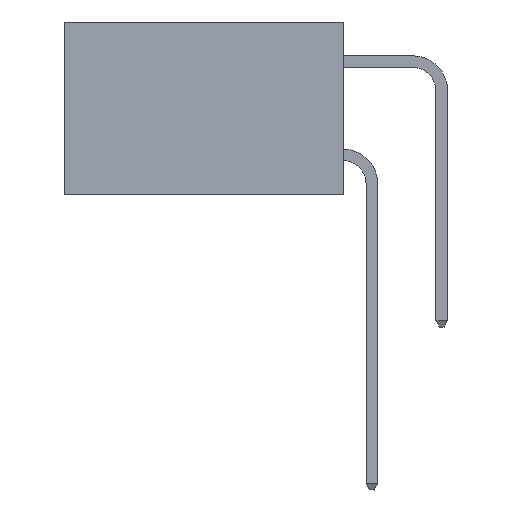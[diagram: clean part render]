
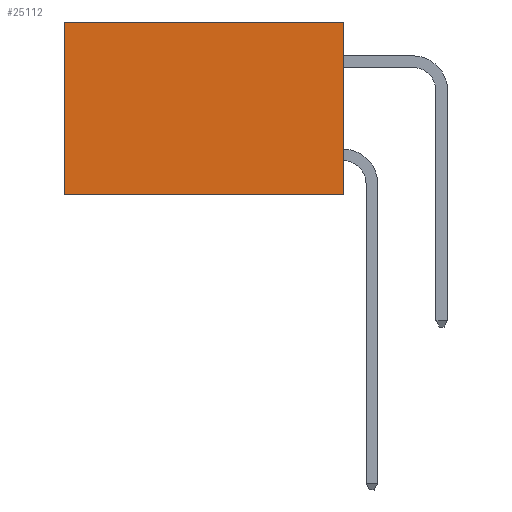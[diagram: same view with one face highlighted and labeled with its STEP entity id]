
A CAD part, left-side view. The second image highlights one B-rep face of the part: STEP entity #25112.
In plain terms, the highlighted planar face has unit normal (-1, 0, 0).
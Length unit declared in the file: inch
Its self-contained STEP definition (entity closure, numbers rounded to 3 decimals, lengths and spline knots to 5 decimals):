
#153 = CARTESIAN_POINT ( 'NONE',  ( 0.298, 0.6, 0. ) ) ;
#1627 = PLANE ( 'NONE',  #24655 ) ;
#2606 = EDGE_CURVE ( 'NONE', #22275, #15814, #2981, .T. ) ;
#2981 = LINE ( 'NONE', #22078, #21465 ) ;
#2990 = ORIENTED_EDGE ( 'NONE', *, *, #2606, .F. ) ;
#5675 = VECTOR ( 'NONE', #22735, 39.37008 ) ;
#6213 = DIRECTION ( 'NONE',  ( 0., 0., -1. ) ) ;
#7237 = CARTESIAN_POINT ( 'NONE',  ( 0.298, 0., -0.37 ) ) ;
#8077 = ORIENTED_EDGE ( 'NONE', *, *, #19435, .T. ) ;
#10208 = FACE_OUTER_BOUND ( 'NONE', #11459, .T. ) ;
#11322 = CARTESIAN_POINT ( 'NONE',  ( 0.298, 0., -0.37 ) ) ;
#11459 = EDGE_LOOP ( 'NONE', ( #8077, #19442, #2990, #21343 ) ) ;
#12739 = VECTOR ( 'NONE', #13634, 39.37008 ) ;
#13634 = DIRECTION ( 'NONE',  ( 0., 0., -1. ) ) ;
#15166 = VERTEX_POINT ( 'NONE', #15851 ) ;
#15814 = VERTEX_POINT ( 'NONE', #11322 ) ;
#15851 = CARTESIAN_POINT ( 'NONE',  ( 0.298, 0.6, 0. ) ) ;
#17306 = CARTESIAN_POINT ( 'NONE',  ( 0.298, 0., 0. ) ) ;
#18606 = LINE ( 'NONE', #153, #12739 ) ;
#19435 = EDGE_CURVE ( 'NONE', #15166, #27762, #18606, .T. ) ;
#19442 = ORIENTED_EDGE ( 'NONE', *, *, #19516, .F. ) ;
#19486 = DIRECTION ( 'NONE',  ( 1., 0., 0. ) ) ;
#19516 = EDGE_CURVE ( 'NONE', #15814, #27762, #22402, .T. ) ;
#20517 = CARTESIAN_POINT ( 'NONE',  ( 0.298, 0., 0. ) ) ;
#21343 = ORIENTED_EDGE ( 'NONE', *, *, #23922, .T. ) ;
#21465 = VECTOR ( 'NONE', #21992, 39.37008 ) ;
#21712 = VECTOR ( 'NONE', #27067, 39.37008 ) ;
#21992 = DIRECTION ( 'NONE',  ( 0., 0., -1. ) ) ;
#22078 = CARTESIAN_POINT ( 'NONE',  ( 0.298, 0., 0. ) ) ;
#22275 = VERTEX_POINT ( 'NONE', #23309 ) ;
#22402 = LINE ( 'NONE', #7237, #21712 ) ;
#22735 = DIRECTION ( 'NONE',  ( 0., 1., 0. ) ) ;
#23309 = CARTESIAN_POINT ( 'NONE',  ( 0.298, 0., 0. ) ) ;
#23372 = LINE ( 'NONE', #20517, #5675 ) ;
#23922 = EDGE_CURVE ( 'NONE', #22275, #15166, #23372, .T. ) ;
#24129 = CARTESIAN_POINT ( 'NONE',  ( 0.298, 0.6, -0.37 ) ) ;
#24655 = AXIS2_PLACEMENT_3D ( 'NONE', #17306, #19486, #6213 ) ;
#25112 = ADVANCED_FACE ( 'NONE', ( #10208 ), #1627, .F. ) ;
#27067 = DIRECTION ( 'NONE',  ( 0., 1., 0. ) ) ;
#27762 = VERTEX_POINT ( 'NONE', #24129 ) ;
